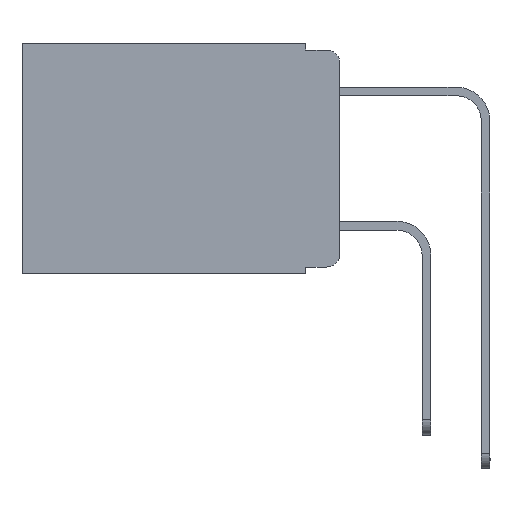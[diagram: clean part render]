
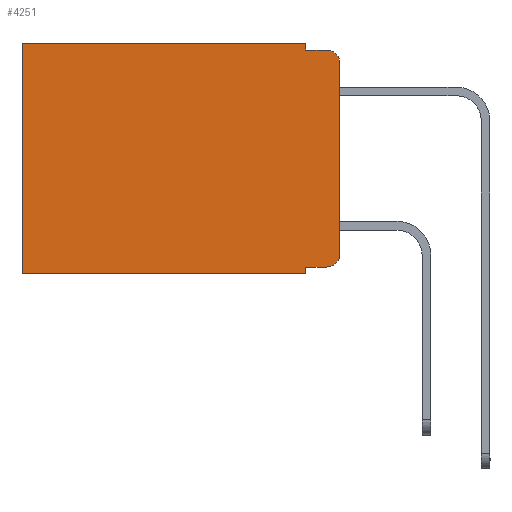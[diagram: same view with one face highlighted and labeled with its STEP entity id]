
A CAD part, left-side view. The second image highlights one B-rep face of the part: STEP entity #4251.
In plain terms, the highlighted planar face has unit normal (-1, 0, 0).
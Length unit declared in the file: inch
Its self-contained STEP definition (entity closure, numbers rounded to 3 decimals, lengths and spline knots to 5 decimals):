
#24 = CIRCLE ( 'NONE', #7406, 0.02 ) ;
#60 = DIRECTION ( 'NONE',  ( -1., 0., 0. ) ) ;
#114 = CARTESIAN_POINT ( 'NONE',  ( 0.298, 0., 0. ) ) ;
#875 = LINE ( 'NONE', #114, #12619 ) ;
#982 = LINE ( 'NONE', #12489, #6991 ) ;
#1032 = DIRECTION ( 'NONE',  ( 0., 0., -1. ) ) ;
#1194 = VERTEX_POINT ( 'NONE', #4343 ) ;
#1246 = VERTEX_POINT ( 'NONE', #11054 ) ;
#1445 = VECTOR ( 'NONE', #10108, 39.37008 ) ;
#1483 = CARTESIAN_POINT ( 'NONE',  ( 0.298, 0.051, 0. ) ) ;
#1550 = EDGE_CURVE ( 'NONE', #1246, #1194, #10882, .T. ) ;
#1787 = ORIENTED_EDGE ( 'NONE', *, *, #12797, .F. ) ;
#1842 = EDGE_CURVE ( 'NONE', #6636, #8400, #12767, .T. ) ;
#2150 = EDGE_CURVE ( 'NONE', #6330, #7577, #12290, .T. ) ;
#2365 = DIRECTION ( 'NONE',  ( 0., 1., 0. ) ) ;
#2584 = CARTESIAN_POINT ( 'NONE',  ( 0.298, 0.473, 0. ) ) ;
#2587 = DIRECTION ( 'NONE',  ( 0., 0., -1. ) ) ;
#2733 = CARTESIAN_POINT ( 'NONE',  ( 0.298, 0.051, 0. ) ) ;
#3115 = ORIENTED_EDGE ( 'NONE', *, *, #4846, .T. ) ;
#3475 = LINE ( 'NONE', #2733, #9716 ) ;
#3794 = VERTEX_POINT ( 'NONE', #2584 ) ;
#4139 = ORIENTED_EDGE ( 'NONE', *, *, #1842, .T. ) ;
#4251 = ADVANCED_FACE ( 'NONE', ( #6064 ), #4657, .F. ) ;
#4343 = CARTESIAN_POINT ( 'NONE',  ( 0.298, 0.473, -0.343 ) ) ;
#4657 = PLANE ( 'NONE',  #6842 ) ;
#4728 = DIRECTION ( 'NONE',  ( 1., 0., 0. ) ) ;
#4846 = EDGE_CURVE ( 'NONE', #6330, #3794, #875, .T. ) ;
#4977 = EDGE_CURVE ( 'NONE', #6636, #1246, #3475, .T. ) ;
#5070 = ORIENTED_EDGE ( 'NONE', *, *, #1550, .F. ) ;
#5356 = CARTESIAN_POINT ( 'NONE',  ( 0.298, 0.02, -0.03 ) ) ;
#5505 = CARTESIAN_POINT ( 'NONE',  ( 0.298, 0., -0.03 ) ) ;
#5540 = CARTESIAN_POINT ( 'NONE',  ( 0.298, 0.051, -0.333 ) ) ;
#5899 = VERTEX_POINT ( 'NONE', #10398 ) ;
#6064 = FACE_OUTER_BOUND ( 'NONE', #9661, .T. ) ;
#6330 = VERTEX_POINT ( 'NONE', #1483 ) ;
#6487 = LINE ( 'NONE', #12340, #11784 ) ;
#6517 = CIRCLE ( 'NONE', #13466, 0.02 ) ;
#6610 = CARTESIAN_POINT ( 'NONE',  ( 0.298, 0., 0. ) ) ;
#6636 = VERTEX_POINT ( 'NONE', #5540 ) ;
#6842 = AXIS2_PLACEMENT_3D ( 'NONE', #14069, #4728, #9205 ) ;
#6991 = VECTOR ( 'NONE', #11276, 39.37008 ) ;
#7406 = AXIS2_PLACEMENT_3D ( 'NONE', #10229, #60, #9020 ) ;
#7490 = DIRECTION ( 'NONE',  ( 0., 1., 0. ) ) ;
#7577 = VERTEX_POINT ( 'NONE', #13207 ) ;
#7604 = EDGE_CURVE ( 'NONE', #10311, #5899, #14625, .T. ) ;
#7836 = VECTOR ( 'NONE', #10437, 39.37008 ) ;
#8400 = VERTEX_POINT ( 'NONE', #10563 ) ;
#8576 = VECTOR ( 'NONE', #1032, 39.37008 ) ;
#8641 = VECTOR ( 'NONE', #7490, 39.37008 ) ;
#8762 = CARTESIAN_POINT ( 'NONE',  ( 0.298, 0.051, 0. ) ) ;
#8805 = DIRECTION ( 'NONE',  ( -1., 0., 0. ) ) ;
#9020 = DIRECTION ( 'NONE',  ( 0., 0., -1. ) ) ;
#9205 = DIRECTION ( 'NONE',  ( 0., 0., -1. ) ) ;
#9494 = CARTESIAN_POINT ( 'NONE',  ( 0.298, 0.02, -0.01 ) ) ;
#9661 = EDGE_LOOP ( 'NONE', ( #14634, #13331, #1787, #13926, #3115, #10957, #5070, #13000, #4139, #11740 ) ) ;
#9716 = VECTOR ( 'NONE', #2587, 39.37008 ) ;
#10108 = DIRECTION ( 'NONE',  ( 0., 0., -1. ) ) ;
#10123 = VERTEX_POINT ( 'NONE', #9494 ) ;
#10160 = DIRECTION ( 'NONE',  ( 0., 0., -1. ) ) ;
#10229 = CARTESIAN_POINT ( 'NONE',  ( 0.298, 0.02, -0.313 ) ) ;
#10311 = VERTEX_POINT ( 'NONE', #5505 ) ;
#10387 = EDGE_CURVE ( 'NONE', #8400, #5899, #24, .T. ) ;
#10398 = CARTESIAN_POINT ( 'NONE',  ( 0.298, 0., -0.313 ) ) ;
#10437 = DIRECTION ( 'NONE',  ( 0., -1., 0. ) ) ;
#10563 = CARTESIAN_POINT ( 'NONE',  ( 0.298, 0.02, -0.333 ) ) ;
#10882 = LINE ( 'NONE', #14318, #8641 ) ;
#10957 = ORIENTED_EDGE ( 'NONE', *, *, #11816, .T. ) ;
#10973 = DIRECTION ( 'NONE',  ( 0., -1., 0. ) ) ;
#11054 = CARTESIAN_POINT ( 'NONE',  ( 0.298, 0.051, -0.343 ) ) ;
#11276 = DIRECTION ( 'NONE',  ( 0., 0., -1. ) ) ;
#11552 = CARTESIAN_POINT ( 'NONE',  ( 0.298, 0.051, -0.333 ) ) ;
#11740 = ORIENTED_EDGE ( 'NONE', *, *, #10387, .T. ) ;
#11784 = VECTOR ( 'NONE', #10973, 39.37008 ) ;
#11816 = EDGE_CURVE ( 'NONE', #3794, #1194, #982, .T. ) ;
#12290 = LINE ( 'NONE', #8762, #1445 ) ;
#12340 = CARTESIAN_POINT ( 'NONE',  ( 0.298, 0.051, -0.01 ) ) ;
#12489 = CARTESIAN_POINT ( 'NONE',  ( 0.298, 0.473, 0. ) ) ;
#12619 = VECTOR ( 'NONE', #2365, 39.37008 ) ;
#12767 = LINE ( 'NONE', #11552, #7836 ) ;
#12797 = EDGE_CURVE ( 'NONE', #7577, #10123, #6487, .T. ) ;
#12858 = EDGE_CURVE ( 'NONE', #10311, #10123, #6517, .T. ) ;
#13000 = ORIENTED_EDGE ( 'NONE', *, *, #4977, .F. ) ;
#13207 = CARTESIAN_POINT ( 'NONE',  ( 0.298, 0.051, -0.01 ) ) ;
#13331 = ORIENTED_EDGE ( 'NONE', *, *, #12858, .T. ) ;
#13466 = AXIS2_PLACEMENT_3D ( 'NONE', #5356, #8805, #10160 ) ;
#13926 = ORIENTED_EDGE ( 'NONE', *, *, #2150, .F. ) ;
#14069 = CARTESIAN_POINT ( 'NONE',  ( 0.298, 0., 0. ) ) ;
#14318 = CARTESIAN_POINT ( 'NONE',  ( 0.298, 0., -0.343 ) ) ;
#14625 = LINE ( 'NONE', #6610, #8576 ) ;
#14634 = ORIENTED_EDGE ( 'NONE', *, *, #7604, .F. ) ;
